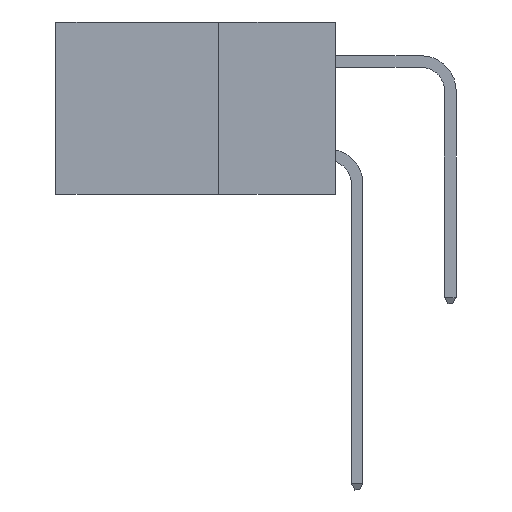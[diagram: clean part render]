
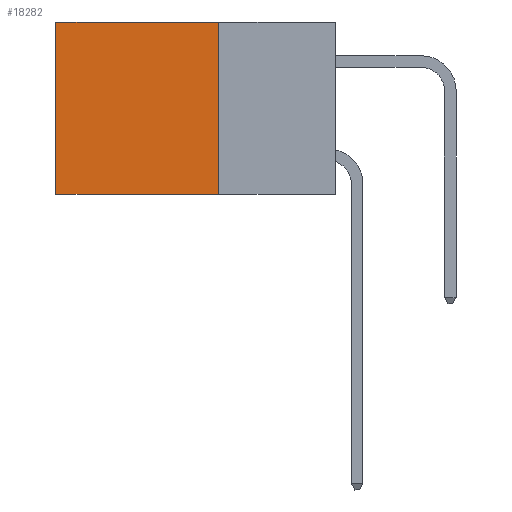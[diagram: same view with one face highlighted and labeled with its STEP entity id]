
A CAD part, left-side view. The second image highlights one B-rep face of the part: STEP entity #18282.
In plain terms, the highlighted planar face has unit normal (-1, 0, 0).
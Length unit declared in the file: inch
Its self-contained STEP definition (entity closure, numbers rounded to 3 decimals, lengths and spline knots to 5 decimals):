
#910 = CARTESIAN_POINT ( 'NONE',  ( 0.2875, 0.6, 0. ) ) ;
#1035 = DIRECTION ( 'NONE',  ( 0., 0., -1. ) ) ;
#1551 = CARTESIAN_POINT ( 'NONE',  ( 0.2875, 0.25, -0.37 ) ) ;
#1581 = DIRECTION ( 'NONE',  ( 0., 1., 0. ) ) ;
#2892 = EDGE_CURVE ( 'NONE', #9272, #3683, #11208, .T. ) ;
#3437 = CARTESIAN_POINT ( 'NONE',  ( 0.2875, 0.25, 0. ) ) ;
#3683 = VERTEX_POINT ( 'NONE', #14236 ) ;
#4722 = VECTOR ( 'NONE', #1581, 39.37008 ) ;
#4741 = CARTESIAN_POINT ( 'NONE',  ( 0.2875, 0.25, 0. ) ) ;
#5940 = ORIENTED_EDGE ( 'NONE', *, *, #27636, .F. ) ;
#8620 = VERTEX_POINT ( 'NONE', #1551 ) ;
#9272 = VERTEX_POINT ( 'NONE', #910 ) ;
#10416 = VECTOR ( 'NONE', #27265, 39.37008 ) ;
#10658 = EDGE_CURVE ( 'NONE', #22357, #9272, #25552, .T. ) ;
#11208 = LINE ( 'NONE', #23629, #11892 ) ;
#11892 = VECTOR ( 'NONE', #28260, 39.37008 ) ;
#12599 = VECTOR ( 'NONE', #25643, 39.37008 ) ;
#12734 = EDGE_LOOP ( 'NONE', ( #27719, #5940, #27860, #16031 ) ) ;
#12898 = CARTESIAN_POINT ( 'NONE',  ( 0.2875, 0.25, -0.37 ) ) ;
#14236 = CARTESIAN_POINT ( 'NONE',  ( 0.2875, 0.6, -0.37 ) ) ;
#16031 = ORIENTED_EDGE ( 'NONE', *, *, #10658, .T. ) ;
#18223 = LINE ( 'NONE', #20940, #12599 ) ;
#18282 = ADVANCED_FACE ( 'NONE', ( #20491 ), #23422, .F. ) ;
#19223 = DIRECTION ( 'NONE',  ( 1., 0., 0. ) ) ;
#20491 = FACE_OUTER_BOUND ( 'NONE', #12734, .T. ) ;
#20940 = CARTESIAN_POINT ( 'NONE',  ( 0.2875, 0.25, 0. ) ) ;
#22242 = AXIS2_PLACEMENT_3D ( 'NONE', #3437, #19223, #1035 ) ;
#22357 = VERTEX_POINT ( 'NONE', #23652 ) ;
#23422 = PLANE ( 'NONE',  #22242 ) ;
#23629 = CARTESIAN_POINT ( 'NONE',  ( 0.2875, 0.6, 0. ) ) ;
#23652 = CARTESIAN_POINT ( 'NONE',  ( 0.2875, 0.25, 0. ) ) ;
#25552 = LINE ( 'NONE', #4741, #10416 ) ;
#25643 = DIRECTION ( 'NONE',  ( 0., 0., -1. ) ) ;
#27265 = DIRECTION ( 'NONE',  ( 0., 1., 0. ) ) ;
#27636 = EDGE_CURVE ( 'NONE', #8620, #3683, #28790, .T. ) ;
#27719 = ORIENTED_EDGE ( 'NONE', *, *, #2892, .T. ) ;
#27860 = ORIENTED_EDGE ( 'NONE', *, *, #28773, .F. ) ;
#28260 = DIRECTION ( 'NONE',  ( 0., 0., -1. ) ) ;
#28773 = EDGE_CURVE ( 'NONE', #22357, #8620, #18223, .T. ) ;
#28790 = LINE ( 'NONE', #12898, #4722 ) ;
